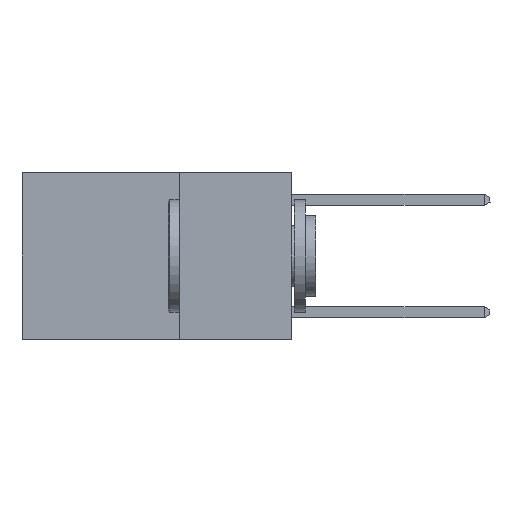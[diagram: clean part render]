
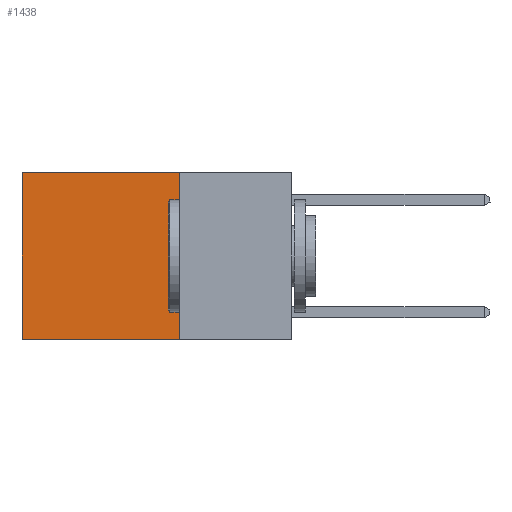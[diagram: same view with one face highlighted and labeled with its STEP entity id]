
A CAD part, left-side view. The second image highlights one B-rep face of the part: STEP entity #1438.
In plain terms, the highlighted planar face has unit normal (-1, 0, 0).
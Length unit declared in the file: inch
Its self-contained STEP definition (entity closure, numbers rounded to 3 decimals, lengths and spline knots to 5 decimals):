
#526 = VERTEX_POINT ( 'NONE', #7606 ) ;
#752 = DIRECTION ( 'NONE',  ( 0., 0., -1. ) ) ;
#1438 = ADVANCED_FACE ( 'NONE', ( #2034 ), #2423, .F. ) ;
#1646 = EDGE_CURVE ( 'NONE', #2086, #3216, #8810, .T. ) ;
#1934 = LINE ( 'NONE', #7933, #10713 ) ;
#2034 = FACE_OUTER_BOUND ( 'NONE', #4623, .T. ) ;
#2086 = VERTEX_POINT ( 'NONE', #4372 ) ;
#2335 = VECTOR ( 'NONE', #9633, 39.37008 ) ;
#2423 = PLANE ( 'NONE',  #3656 ) ;
#3216 = VERTEX_POINT ( 'NONE', #9417 ) ;
#3591 = ORIENTED_EDGE ( 'NONE', *, *, #6935, .T. ) ;
#3656 = AXIS2_PLACEMENT_3D ( 'NONE', #8351, #6548, #752 ) ;
#4372 = CARTESIAN_POINT ( 'NONE',  ( 0.2625, 0.25, 0. ) ) ;
#4393 = EDGE_CURVE ( 'NONE', #526, #7423, #4622, .T. ) ;
#4457 = ORIENTED_EDGE ( 'NONE', *, *, #1646, .F. ) ;
#4546 = DIRECTION ( 'NONE',  ( 0., 0., -1. ) ) ;
#4622 = LINE ( 'NONE', #6241, #5163 ) ;
#4623 = EDGE_LOOP ( 'NONE', ( #6733, #5993, #4457, #3591 ) ) ;
#4838 = DIRECTION ( 'NONE',  ( 0., 0., -1. ) ) ;
#5163 = VECTOR ( 'NONE', #4546, 39.37008 ) ;
#5476 = CARTESIAN_POINT ( 'NONE',  ( 0.2625, 0.25, 0. ) ) ;
#5993 = ORIENTED_EDGE ( 'NONE', *, *, #6590, .F. ) ;
#6241 = CARTESIAN_POINT ( 'NONE',  ( 0.2625, 0.6, 0. ) ) ;
#6548 = DIRECTION ( 'NONE',  ( 1., 0., 0. ) ) ;
#6590 = EDGE_CURVE ( 'NONE', #3216, #7423, #1934, .T. ) ;
#6733 = ORIENTED_EDGE ( 'NONE', *, *, #4393, .T. ) ;
#6935 = EDGE_CURVE ( 'NONE', #2086, #526, #10849, .T. ) ;
#7423 = VERTEX_POINT ( 'NONE', #9206 ) ;
#7606 = CARTESIAN_POINT ( 'NONE',  ( 0.2625, 0.6, 0. ) ) ;
#7933 = CARTESIAN_POINT ( 'NONE',  ( 0.2625, 0.25, -0.37 ) ) ;
#8351 = CARTESIAN_POINT ( 'NONE',  ( 0.2625, 0.25, 0. ) ) ;
#8810 = LINE ( 'NONE', #5476, #10040 ) ;
#8824 = CARTESIAN_POINT ( 'NONE',  ( 0.2625, 0.25, 0. ) ) ;
#9206 = CARTESIAN_POINT ( 'NONE',  ( 0.2625, 0.6, -0.37 ) ) ;
#9417 = CARTESIAN_POINT ( 'NONE',  ( 0.2625, 0.25, -0.37 ) ) ;
#9633 = DIRECTION ( 'NONE',  ( 0., 1., 0. ) ) ;
#9731 = DIRECTION ( 'NONE',  ( 0., 1., 0. ) ) ;
#10040 = VECTOR ( 'NONE', #4838, 39.37008 ) ;
#10713 = VECTOR ( 'NONE', #9731, 39.37008 ) ;
#10849 = LINE ( 'NONE', #8824, #2335 ) ;
